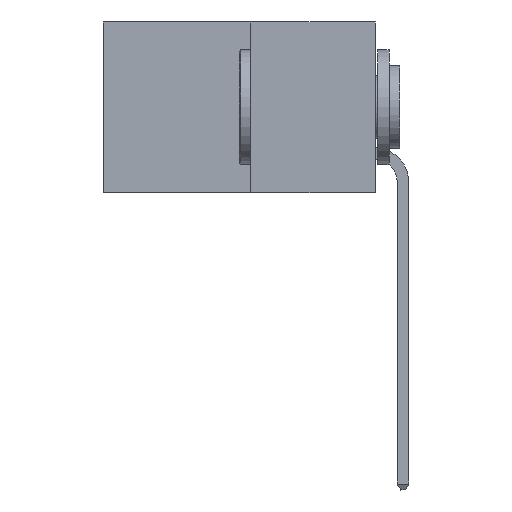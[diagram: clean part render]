
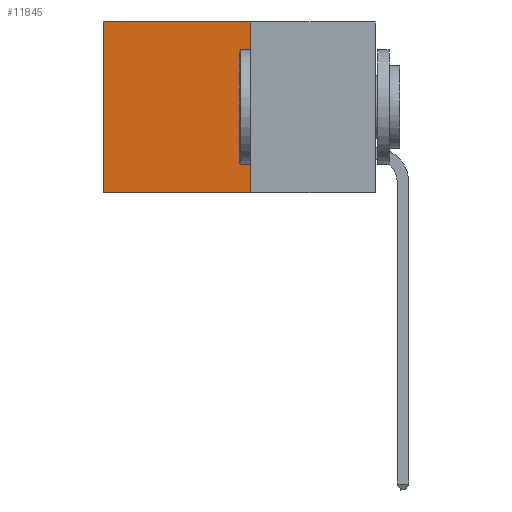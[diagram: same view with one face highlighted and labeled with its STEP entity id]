
A CAD part, left-side view. The second image highlights one B-rep face of the part: STEP entity #11845.
In plain terms, the highlighted planar face has unit normal (-1, 0, 0).
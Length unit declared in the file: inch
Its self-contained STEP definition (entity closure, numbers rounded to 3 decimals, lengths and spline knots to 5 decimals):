
#86 = VERTEX_POINT ( 'NONE', #2106 ) ;
#498 = VECTOR ( 'NONE', #14291, 39.37008 ) ;
#1198 = ORIENTED_EDGE ( 'NONE', *, *, #12784, .F. ) ;
#1219 = AXIS2_PLACEMENT_3D ( 'NONE', #8616, #13290, #6212 ) ;
#1269 = VERTEX_POINT ( 'NONE', #9911 ) ;
#1804 = EDGE_CURVE ( 'NONE', #10389, #13278, #2469, .T. ) ;
#2060 = VECTOR ( 'NONE', #7236, 39.37008 ) ;
#2106 = CARTESIAN_POINT ( 'NONE',  ( 0.277, 0.27, -0.37 ) ) ;
#2425 = EDGE_CURVE ( 'NONE', #13278, #1269, #5283, .T. ) ;
#2469 = LINE ( 'NONE', #6377, #5313 ) ;
#3766 = ORIENTED_EDGE ( 'NONE', *, *, #14445, .F. ) ;
#3921 = CARTESIAN_POINT ( 'NONE',  ( 0.277, 0.27, 0. ) ) ;
#5092 = LINE ( 'NONE', #15331, #498 ) ;
#5283 = LINE ( 'NONE', #7411, #2060 ) ;
#5313 = VECTOR ( 'NONE', #6831, 39.37008 ) ;
#5432 = VECTOR ( 'NONE', #8060, 39.37008 ) ;
#5814 = LINE ( 'NONE', #6799, #5432 ) ;
#5972 = ORIENTED_EDGE ( 'NONE', *, *, #1804, .T. ) ;
#6212 = DIRECTION ( 'NONE',  ( 0., 0., -1. ) ) ;
#6377 = CARTESIAN_POINT ( 'NONE',  ( 0.277, 0.27, 0. ) ) ;
#6391 = FACE_OUTER_BOUND ( 'NONE', #13060, .T. ) ;
#6799 = CARTESIAN_POINT ( 'NONE',  ( 0.277, 0.27, -0.37 ) ) ;
#6831 = DIRECTION ( 'NONE',  ( 0., 1., 0. ) ) ;
#7236 = DIRECTION ( 'NONE',  ( 0., 0., -1. ) ) ;
#7411 = CARTESIAN_POINT ( 'NONE',  ( 0.277, 0.59, -0.37 ) ) ;
#8060 = DIRECTION ( 'NONE',  ( 0., 1., 0. ) ) ;
#8616 = CARTESIAN_POINT ( 'NONE',  ( 0.277, 0.27, -0.37 ) ) ;
#9911 = CARTESIAN_POINT ( 'NONE',  ( 0.277, 0.59, -0.37 ) ) ;
#10389 = VERTEX_POINT ( 'NONE', #3921 ) ;
#11845 = ADVANCED_FACE ( 'NONE', ( #6391 ), #12104, .F. ) ;
#12104 = PLANE ( 'NONE',  #1219 ) ;
#12784 = EDGE_CURVE ( 'NONE', #86, #1269, #5814, .T. ) ;
#13060 = EDGE_LOOP ( 'NONE', ( #14320, #1198, #3766, #5972 ) ) ;
#13278 = VERTEX_POINT ( 'NONE', #14859 ) ;
#13290 = DIRECTION ( 'NONE',  ( 1., 0., 0. ) ) ;
#14291 = DIRECTION ( 'NONE',  ( 0., 0., -1. ) ) ;
#14320 = ORIENTED_EDGE ( 'NONE', *, *, #2425, .T. ) ;
#14445 = EDGE_CURVE ( 'NONE', #10389, #86, #5092, .T. ) ;
#14859 = CARTESIAN_POINT ( 'NONE',  ( 0.277, 0.59, 0. ) ) ;
#15331 = CARTESIAN_POINT ( 'NONE',  ( 0.277, 0.27, -0.37 ) ) ;
